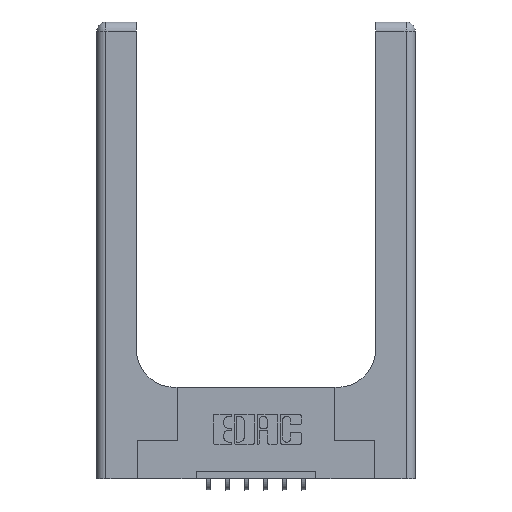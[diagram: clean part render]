
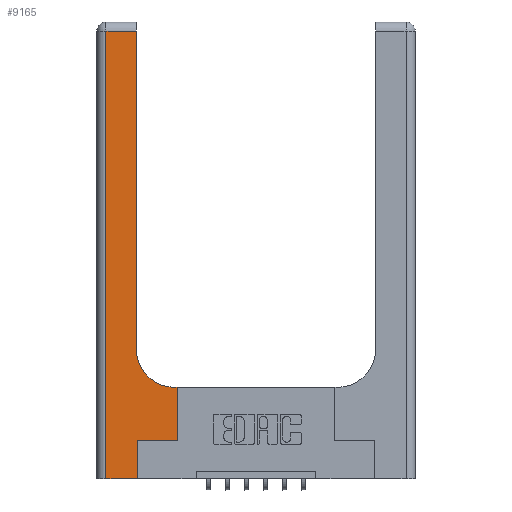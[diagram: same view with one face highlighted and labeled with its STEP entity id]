
A CAD part, top view. The second image highlights one B-rep face of the part: STEP entity #9165.
In plain terms, the highlighted planar face has unit normal (0, 0, 1).
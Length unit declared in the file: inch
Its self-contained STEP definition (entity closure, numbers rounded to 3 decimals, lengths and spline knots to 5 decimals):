
#18 = VECTOR ( 'NONE', #14265, 39.37008 ) ;
#63 = CARTESIAN_POINT ( 'NONE',  ( 0.06, 3., 0.37 ) ) ;
#251 = VERTEX_POINT ( 'NONE', #14281 ) ;
#600 = EDGE_CURVE ( 'NONE', #9784, #10032, #11226, .T. ) ;
#678 = CARTESIAN_POINT ( 'NONE',  ( 0.51, 0.6, 0.37 ) ) ;
#1009 = EDGE_LOOP ( 'NONE', ( #10267, #13014, #4190, #7731, #11933, #8092, #6306, #13557, #12062 ) ) ;
#1065 = VERTEX_POINT ( 'NONE', #9673 ) ;
#1483 = VECTOR ( 'NONE', #9979, 39.37008 ) ;
#1569 = LINE ( 'NONE', #9286, #11568 ) ;
#1869 = FACE_OUTER_BOUND ( 'NONE', #1009, .T. ) ;
#2095 = LINE ( 'NONE', #10919, #18 ) ;
#2260 = CARTESIAN_POINT ( 'NONE',  ( 0.528, 0.6, 0.37 ) ) ;
#2447 = CIRCLE ( 'NONE', #13311, 0.25 ) ;
#2835 = LINE ( 'NONE', #4998, #3062 ) ;
#3062 = VECTOR ( 'NONE', #11739, 39.37008 ) ;
#3207 = EDGE_CURVE ( 'NONE', #11044, #14130, #2447, .T. ) ;
#3239 = PLANE ( 'NONE',  #12476 ) ;
#3358 = DIRECTION ( 'NONE',  ( 0., -1., 0. ) ) ;
#3383 = VERTEX_POINT ( 'NONE', #2260 ) ;
#3775 = VECTOR ( 'NONE', #4687, 39.37008 ) ;
#4088 = DIRECTION ( 'NONE',  ( 0., 0., -1. ) ) ;
#4112 = CARTESIAN_POINT ( 'NONE',  ( 0., 3., 0.37 ) ) ;
#4190 = ORIENTED_EDGE ( 'NONE', *, *, #4868, .T. ) ;
#4687 = DIRECTION ( 'NONE',  ( 0., 1., 0. ) ) ;
#4796 = CARTESIAN_POINT ( 'NONE',  ( 0.26, 0.85, 0.37 ) ) ;
#4868 = EDGE_CURVE ( 'NONE', #10032, #1065, #13400, .T. ) ;
#4998 = CARTESIAN_POINT ( 'NONE',  ( 0., 0., 0.37 ) ) ;
#5650 = CARTESIAN_POINT ( 'NONE',  ( 0.26, 3., 0.37 ) ) ;
#5764 = LINE ( 'NONE', #10163, #3775 ) ;
#6304 = DIRECTION ( 'NONE',  ( 1., 0., 0. ) ) ;
#6306 = ORIENTED_EDGE ( 'NONE', *, *, #7320, .T. ) ;
#6634 = CARTESIAN_POINT ( 'NONE',  ( 0.26, 2.94, 0.37 ) ) ;
#6658 = DIRECTION ( 'NONE',  ( 0., 1., 0. ) ) ;
#7320 = EDGE_CURVE ( 'NONE', #11157, #3383, #2095, .T. ) ;
#7545 = CARTESIAN_POINT ( 'NONE',  ( 0.51, 0.85, 0.37 ) ) ;
#7731 = ORIENTED_EDGE ( 'NONE', *, *, #14231, .T. ) ;
#7902 = VECTOR ( 'NONE', #6658, 39.37008 ) ;
#8092 = ORIENTED_EDGE ( 'NONE', *, *, #10726, .T. ) ;
#8185 = CARTESIAN_POINT ( 'NONE',  ( 0.26, 0.6, 0.37 ) ) ;
#8946 = VECTOR ( 'NONE', #3358, 39.37008 ) ;
#9165 = ADVANCED_FACE ( 'NONE', ( #1869 ), #3239, .F. ) ;
#9286 = CARTESIAN_POINT ( 'NONE',  ( 0.265, 0.25, 0.37 ) ) ;
#9673 = CARTESIAN_POINT ( 'NONE',  ( 0.06, 0., 0.37 ) ) ;
#9679 = CARTESIAN_POINT ( 'NONE',  ( 0.528, 0.25, 0.37 ) ) ;
#9784 = VERTEX_POINT ( 'NONE', #6634 ) ;
#9979 = DIRECTION ( 'NONE',  ( -1., 0., 0. ) ) ;
#10032 = VERTEX_POINT ( 'NONE', #10826 ) ;
#10044 = CARTESIAN_POINT ( 'NONE',  ( 0., 2.94, 0.37 ) ) ;
#10163 = CARTESIAN_POINT ( 'NONE',  ( 0.265, 0., 0.37 ) ) ;
#10267 = ORIENTED_EDGE ( 'NONE', *, *, #12147, .T. ) ;
#10662 = CARTESIAN_POINT ( 'NONE',  ( 0.265, 0., 0.37 ) ) ;
#10726 = EDGE_CURVE ( 'NONE', #251, #11157, #1569, .T. ) ;
#10826 = CARTESIAN_POINT ( 'NONE',  ( 0.06, 2.94, 0.37 ) ) ;
#10919 = CARTESIAN_POINT ( 'NONE',  ( 0.528, 0.25, 0.37 ) ) ;
#11044 = VERTEX_POINT ( 'NONE', #678 ) ;
#11157 = VERTEX_POINT ( 'NONE', #9679 ) ;
#11226 = LINE ( 'NONE', #10044, #1483 ) ;
#11320 = DIRECTION ( 'NONE',  ( 1., 0., 0. ) ) ;
#11568 = VECTOR ( 'NONE', #11320, 39.37008 ) ;
#11739 = DIRECTION ( 'NONE',  ( 1., 0., 0. ) ) ;
#11933 = ORIENTED_EDGE ( 'NONE', *, *, #13792, .T. ) ;
#12062 = ORIENTED_EDGE ( 'NONE', *, *, #3207, .T. ) ;
#12147 = EDGE_CURVE ( 'NONE', #14130, #9784, #12262, .T. ) ;
#12251 = EDGE_CURVE ( 'NONE', #3383, #11044, #12547, .T. ) ;
#12262 = LINE ( 'NONE', #5650, #7902 ) ;
#12476 = AXIS2_PLACEMENT_3D ( 'NONE', #4112, #12934, #14176 ) ;
#12547 = LINE ( 'NONE', #8185, #14160 ) ;
#12613 = DIRECTION ( 'NONE',  ( -1., 0., 0. ) ) ;
#12934 = DIRECTION ( 'NONE',  ( 0., 0., -1. ) ) ;
#13014 = ORIENTED_EDGE ( 'NONE', *, *, #600, .T. ) ;
#13049 = VERTEX_POINT ( 'NONE', #10662 ) ;
#13311 = AXIS2_PLACEMENT_3D ( 'NONE', #7545, #4088, #6304 ) ;
#13400 = LINE ( 'NONE', #63, #8946 ) ;
#13557 = ORIENTED_EDGE ( 'NONE', *, *, #12251, .T. ) ;
#13792 = EDGE_CURVE ( 'NONE', #13049, #251, #5764, .T. ) ;
#14130 = VERTEX_POINT ( 'NONE', #4796 ) ;
#14160 = VECTOR ( 'NONE', #12613, 39.37008 ) ;
#14176 = DIRECTION ( 'NONE',  ( -1., 0., 0. ) ) ;
#14231 = EDGE_CURVE ( 'NONE', #1065, #13049, #2835, .T. ) ;
#14265 = DIRECTION ( 'NONE',  ( 0., 1., 0. ) ) ;
#14281 = CARTESIAN_POINT ( 'NONE',  ( 0.265, 0.25, 0.37 ) ) ;
